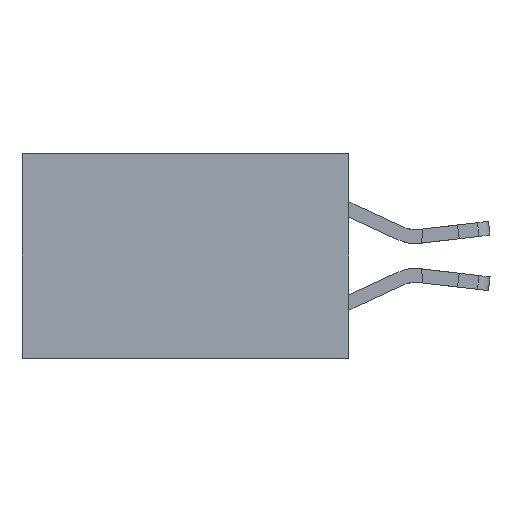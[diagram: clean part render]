
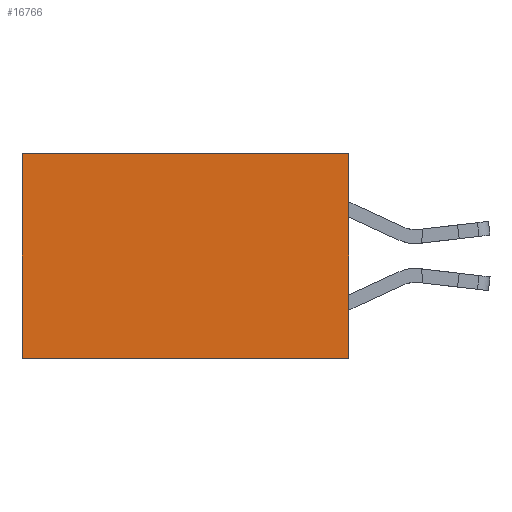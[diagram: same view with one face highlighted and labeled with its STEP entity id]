
A CAD part, left-side view. The second image highlights one B-rep face of the part: STEP entity #16766.
In plain terms, the highlighted planar face has unit normal (-1, 0, 0).
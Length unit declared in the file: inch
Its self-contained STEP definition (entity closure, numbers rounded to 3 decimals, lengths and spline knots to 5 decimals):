
#698 = CARTESIAN_POINT ( 'NONE',  ( 0.277, 0., 0. ) ) ;
#752 = VECTOR ( 'NONE', #2111, 39.37008 ) ;
#1483 = ORIENTED_EDGE ( 'NONE', *, *, #14348, .T. ) ;
#1583 = VERTEX_POINT ( 'NONE', #14207 ) ;
#1593 = CARTESIAN_POINT ( 'NONE',  ( 0.277, 0., -0.37 ) ) ;
#1647 = AXIS2_PLACEMENT_3D ( 'NONE', #14673, #8760, #19031 ) ;
#2111 = DIRECTION ( 'NONE',  ( 0., 1., 0. ) ) ;
#3081 = LINE ( 'NONE', #11872, #14580 ) ;
#3699 = ORIENTED_EDGE ( 'NONE', *, *, #16784, .F. ) ;
#4714 = CARTESIAN_POINT ( 'NONE',  ( 0.277, 0.59, -0.37 ) ) ;
#5723 = CARTESIAN_POINT ( 'NONE',  ( 0.277, 0., -0.37 ) ) ;
#5788 = DIRECTION ( 'NONE',  ( 0., 0., -1. ) ) ;
#5920 = DIRECTION ( 'NONE',  ( 0., 1., 0. ) ) ;
#8282 = EDGE_CURVE ( 'NONE', #16007, #10544, #15791, .T. ) ;
#8463 = ORIENTED_EDGE ( 'NONE', *, *, #14657, .F. ) ;
#8721 = VECTOR ( 'NONE', #5788, 39.37008 ) ;
#8760 = DIRECTION ( 'NONE',  ( 1., 0., 0. ) ) ;
#9151 = FACE_OUTER_BOUND ( 'NONE', #14613, .T. ) ;
#10544 = VERTEX_POINT ( 'NONE', #16821 ) ;
#11043 = ORIENTED_EDGE ( 'NONE', *, *, #8282, .T. ) ;
#11395 = VECTOR ( 'NONE', #18436, 39.37008 ) ;
#11872 = CARTESIAN_POINT ( 'NONE',  ( 0.277, 0., -0.37 ) ) ;
#12683 = LINE ( 'NONE', #5723, #8721 ) ;
#12750 = LINE ( 'NONE', #698, #752 ) ;
#12878 = CARTESIAN_POINT ( 'NONE',  ( 0.277, 0.59, 0. ) ) ;
#14207 = CARTESIAN_POINT ( 'NONE',  ( 0.277, 0., 0. ) ) ;
#14348 = EDGE_CURVE ( 'NONE', #1583, #16007, #12750, .T. ) ;
#14580 = VECTOR ( 'NONE', #5920, 39.37008 ) ;
#14613 = EDGE_LOOP ( 'NONE', ( #11043, #8463, #3699, #1483 ) ) ;
#14657 = EDGE_CURVE ( 'NONE', #19129, #10544, #3081, .T. ) ;
#14673 = CARTESIAN_POINT ( 'NONE',  ( 0.277, 0., -0.37 ) ) ;
#15791 = LINE ( 'NONE', #4714, #11395 ) ;
#16007 = VERTEX_POINT ( 'NONE', #12878 ) ;
#16140 = PLANE ( 'NONE',  #1647 ) ;
#16766 = ADVANCED_FACE ( 'NONE', ( #9151 ), #16140, .F. ) ;
#16784 = EDGE_CURVE ( 'NONE', #1583, #19129, #12683, .T. ) ;
#16821 = CARTESIAN_POINT ( 'NONE',  ( 0.277, 0.59, -0.37 ) ) ;
#18436 = DIRECTION ( 'NONE',  ( 0., 0., -1. ) ) ;
#19031 = DIRECTION ( 'NONE',  ( 0., 0., -1. ) ) ;
#19129 = VERTEX_POINT ( 'NONE', #1593 ) ;
